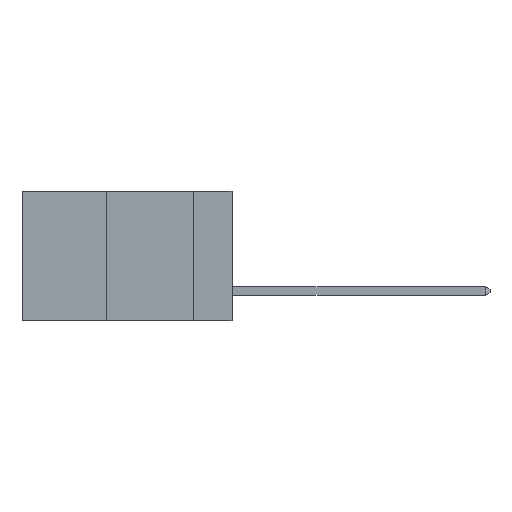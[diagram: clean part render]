
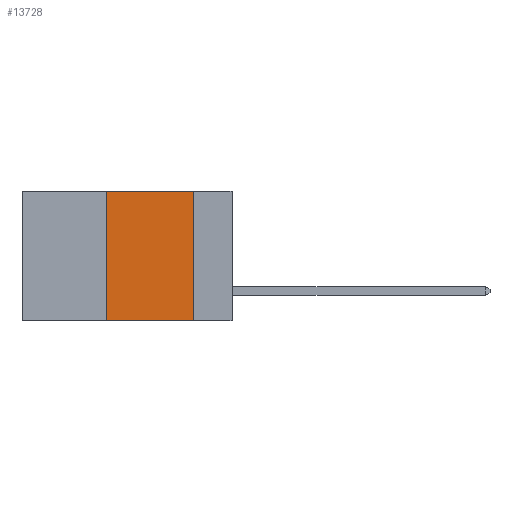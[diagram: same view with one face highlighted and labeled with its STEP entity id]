
A CAD part, left-side view. The second image highlights one B-rep face of the part: STEP entity #13728.
In plain terms, the highlighted planar face has unit normal (-1, 0, 0).
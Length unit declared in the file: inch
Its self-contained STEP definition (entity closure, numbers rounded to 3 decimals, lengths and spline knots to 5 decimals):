
#1647 = DIRECTION ( 'NONE',  ( 0., 0., -1. ) ) ;
#2568 = AXIS2_PLACEMENT_3D ( 'NONE', #7439, #19116, #1647 ) ;
#2735 = LINE ( 'NONE', #3773, #33459 ) ;
#3773 = CARTESIAN_POINT ( 'NONE',  ( 0., 0.6, -0.37 ) ) ;
#4287 = EDGE_LOOP ( 'NONE', ( #36785, #15068, #14412, #21135 ) ) ;
#5428 = EDGE_CURVE ( 'NONE', #17025, #31283, #29558, .T. ) ;
#5715 = CARTESIAN_POINT ( 'NONE',  ( 0., 0.36, 0. ) ) ;
#6969 = CARTESIAN_POINT ( 'NONE',  ( 0., 0.11, 0. ) ) ;
#7439 = CARTESIAN_POINT ( 'NONE',  ( 0., 0.6, 0. ) ) ;
#8146 = FACE_OUTER_BOUND ( 'NONE', #4287, .T. ) ;
#9240 = VECTOR ( 'NONE', #30746, 39.37008 ) ;
#10610 = CARTESIAN_POINT ( 'NONE',  ( 0., 0.36, 0. ) ) ;
#13387 = VECTOR ( 'NONE', #32671, 39.37008 ) ;
#13728 = ADVANCED_FACE ( 'NONE', ( #8146 ), #36184, .F. ) ;
#13930 = LINE ( 'NONE', #35242, #28291 ) ;
#14412 = ORIENTED_EDGE ( 'NONE', *, *, #31597, .F. ) ;
#15068 = ORIENTED_EDGE ( 'NONE', *, *, #30200, .F. ) ;
#15300 = DIRECTION ( 'NONE',  ( 0., -1., 0. ) ) ;
#17025 = VERTEX_POINT ( 'NONE', #6969 ) ;
#18270 = CARTESIAN_POINT ( 'NONE',  ( 0., 0.11, 0. ) ) ;
#19116 = DIRECTION ( 'NONE',  ( 1., 0., 0. ) ) ;
#20968 = CARTESIAN_POINT ( 'NONE',  ( 0., 0.36, -0.37 ) ) ;
#21135 = ORIENTED_EDGE ( 'NONE', *, *, #21592, .T. ) ;
#21592 = EDGE_CURVE ( 'NONE', #24011, #31283, #2735, .T. ) ;
#24011 = VERTEX_POINT ( 'NONE', #20968 ) ;
#24075 = DIRECTION ( 'NONE',  ( 0., -1., 0. ) ) ;
#25801 = VERTEX_POINT ( 'NONE', #5715 ) ;
#28291 = VECTOR ( 'NONE', #15300, 39.37008 ) ;
#29558 = LINE ( 'NONE', #18270, #13387 ) ;
#30200 = EDGE_CURVE ( 'NONE', #25801, #17025, #13930, .T. ) ;
#30746 = DIRECTION ( 'NONE',  ( 0., 0., 1. ) ) ;
#31283 = VERTEX_POINT ( 'NONE', #37027 ) ;
#31331 = LINE ( 'NONE', #10610, #9240 ) ;
#31597 = EDGE_CURVE ( 'NONE', #24011, #25801, #31331, .T. ) ;
#32671 = DIRECTION ( 'NONE',  ( 0., 0., -1. ) ) ;
#33459 = VECTOR ( 'NONE', #24075, 39.37008 ) ;
#35242 = CARTESIAN_POINT ( 'NONE',  ( 0., 0.6, 0. ) ) ;
#36184 = PLANE ( 'NONE',  #2568 ) ;
#36785 = ORIENTED_EDGE ( 'NONE', *, *, #5428, .F. ) ;
#37027 = CARTESIAN_POINT ( 'NONE',  ( 0., 0.11, -0.37 ) ) ;
